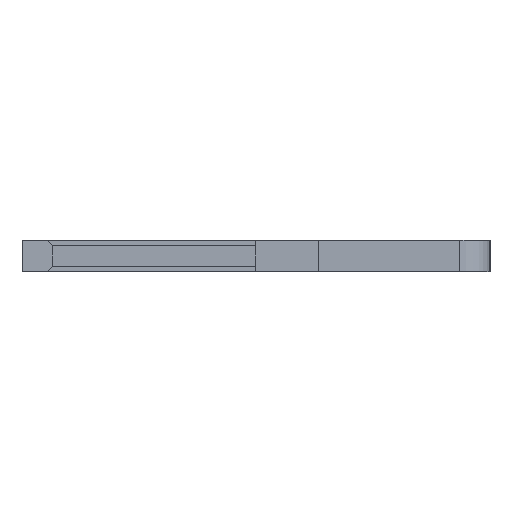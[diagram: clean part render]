
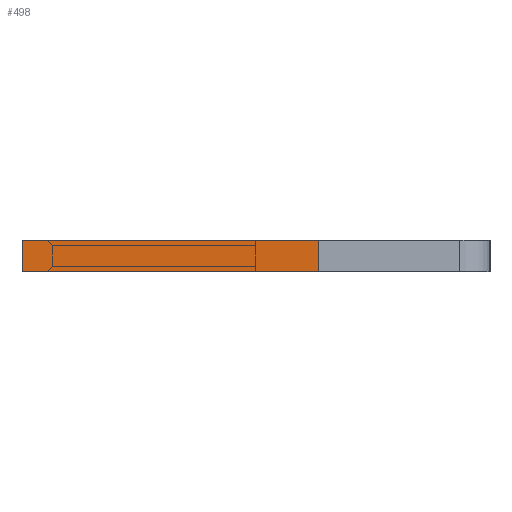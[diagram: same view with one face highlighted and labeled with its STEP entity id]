
A CAD part, left-side view. The second image highlights one B-rep face of the part: STEP entity #498.
In plain terms, the highlighted face is planar.
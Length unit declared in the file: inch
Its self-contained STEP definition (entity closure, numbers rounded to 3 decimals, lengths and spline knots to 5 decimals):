
#10 = CARTESIAN_POINT ( 'NONE',  ( -0.01, 0.15, -0.04 ) ) ;
#146 = VERTEX_POINT ( 'NONE', #3228 ) ;
#237 = LINE ( 'NONE', #10, #2662 ) ;
#495 = CARTESIAN_POINT ( 'NONE',  ( -0.01, 0.15, -0.04 ) ) ;
#498 = ADVANCED_FACE ( 'NONE', ( #1833 ), #1235, .F. ) ;
#501 = LINE ( 'NONE', #918, #3696 ) ;
#544 = DIRECTION ( 'NONE',  ( 1., 0., 0. ) ) ;
#615 = DIRECTION ( 'NONE',  ( -1., 0., 0. ) ) ;
#748 = VERTEX_POINT ( 'NONE', #495 ) ;
#838 = LINE ( 'NONE', #3411, #2868 ) ;
#908 = ORIENTED_EDGE ( 'NONE', *, *, #1067, .T. ) ;
#918 = CARTESIAN_POINT ( 'NONE',  ( 0.01, 0.15, -0.04 ) ) ;
#1067 = EDGE_CURVE ( 'NONE', #146, #4259, #838, .T. ) ;
#1235 = PLANE ( 'NONE',  #4043 ) ;
#1271 = ORIENTED_EDGE ( 'NONE', *, *, #1319, .F. ) ;
#1319 = EDGE_CURVE ( 'NONE', #2779, #748, #501, .T. ) ;
#1398 = ORIENTED_EDGE ( 'NONE', *, *, #2524, .F. ) ;
#1484 = CARTESIAN_POINT ( 'NONE',  ( 0.01, 0.15, -0.04 ) ) ;
#1784 = VECTOR ( 'NONE', #3138, 39.37008 ) ;
#1833 = FACE_OUTER_BOUND ( 'NONE', #3556, .T. ) ;
#2524 = EDGE_CURVE ( 'NONE', #146, #2779, #2718, .T. ) ;
#2661 = CARTESIAN_POINT ( 'NONE',  ( 0.01, 0.15, -0.04 ) ) ;
#2662 = VECTOR ( 'NONE', #4153, 39.37008 ) ;
#2718 = LINE ( 'NONE', #2781, #1784 ) ;
#2778 = CARTESIAN_POINT ( 'NONE',  ( -0.01, -0.04, -0.04 ) ) ;
#2779 = VERTEX_POINT ( 'NONE', #1484 ) ;
#2781 = CARTESIAN_POINT ( 'NONE',  ( 0.01, 0.15, -0.04 ) ) ;
#2868 = VECTOR ( 'NONE', #4421, 39.37008 ) ;
#3138 = DIRECTION ( 'NONE',  ( 0., 1., 0. ) ) ;
#3228 = CARTESIAN_POINT ( 'NONE',  ( 0.01, -0.04, -0.04 ) ) ;
#3411 = CARTESIAN_POINT ( 'NONE',  ( 0.01, -0.04, -0.04 ) ) ;
#3556 = EDGE_LOOP ( 'NONE', ( #3971, #1271, #1398, #908 ) ) ;
#3696 = VECTOR ( 'NONE', #615, 39.37008 ) ;
#3971 = ORIENTED_EDGE ( 'NONE', *, *, #4217, .T. ) ;
#4023 = DIRECTION ( 'NONE',  ( 0., 0., 1. ) ) ;
#4043 = AXIS2_PLACEMENT_3D ( 'NONE', #2661, #4023, #544 ) ;
#4153 = DIRECTION ( 'NONE',  ( 0., 1., 0. ) ) ;
#4217 = EDGE_CURVE ( 'NONE', #4259, #748, #237, .T. ) ;
#4259 = VERTEX_POINT ( 'NONE', #2778 ) ;
#4421 = DIRECTION ( 'NONE',  ( -1., 0., 0. ) ) ;
